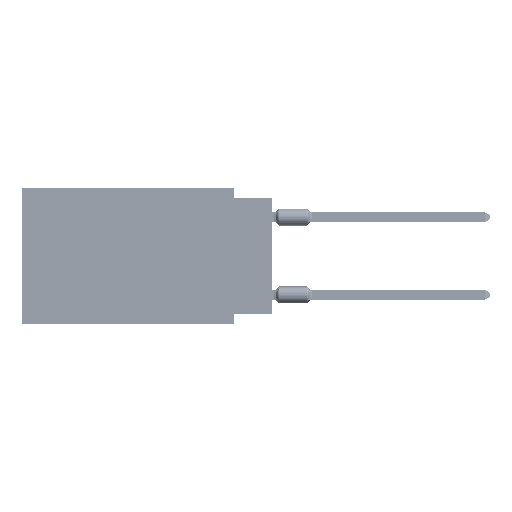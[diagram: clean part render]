
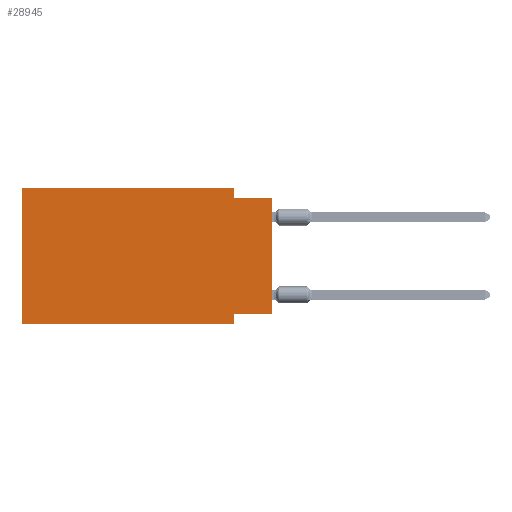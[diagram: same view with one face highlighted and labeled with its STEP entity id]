
A CAD part, left-side view. The second image highlights one B-rep face of the part: STEP entity #28945.
In plain terms, the highlighted planar face has unit normal (-1, 0, 0).
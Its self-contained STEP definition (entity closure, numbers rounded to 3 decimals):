
#859 = FACE_OUTER_BOUND ( 'NONE', #63787, .T. ) ;
#2923 = CARTESIAN_POINT ( 'NONE',  ( 0., 0., -8.255 ) ) ;
#4241 = EDGE_CURVE ( 'NONE', #46899, #16961, #41507, .T. ) ;
#4264 = LINE ( 'NONE', #56788, #30928 ) ;
#4663 = VECTOR ( 'NONE', #31019, 1000. ) ;
#4807 = CARTESIAN_POINT ( 'NONE',  ( 0., 0., -8.255 ) ) ;
#5105 = CARTESIAN_POINT ( 'NONE',  ( 0., 0., -0.635 ) ) ;
#5381 = CARTESIAN_POINT ( 'NONE',  ( 0., 0., 0. ) ) ;
#9938 = VERTEX_POINT ( 'NONE', #48765 ) ;
#11227 = LINE ( 'NONE', #5381, #59317 ) ;
#12024 = VERTEX_POINT ( 'NONE', #26387 ) ;
#13480 = DIRECTION ( 'NONE',  ( 0., -1., 0. ) ) ;
#13601 = ORIENTED_EDGE ( 'NONE', *, *, #71519, .T. ) ;
#14333 = VECTOR ( 'NONE', #43107, 1000. ) ;
#14846 = VECTOR ( 'NONE', #13480, 1000. ) ;
#16961 = VERTEX_POINT ( 'NONE', #5105 ) ;
#18136 = LINE ( 'NONE', #59744, #58381 ) ;
#18648 = VERTEX_POINT ( 'NONE', #25229 ) ;
#19322 = CARTESIAN_POINT ( 'NONE',  ( 0., 0., -0.635 ) ) ;
#19661 = VECTOR ( 'NONE', #68702, 1000. ) ;
#21537 = VERTEX_POINT ( 'NONE', #2923 ) ;
#23590 = DIRECTION ( 'NONE',  ( 0., 0., 1. ) ) ;
#23754 = EDGE_CURVE ( 'NONE', #74258, #9938, #4264, .T. ) ;
#24216 = CARTESIAN_POINT ( 'NONE',  ( 0., 16.383, 0. ) ) ;
#24217 = VERTEX_POINT ( 'NONE', #26371 ) ;
#24594 = PLANE ( 'NONE',  #66621 ) ;
#25229 = CARTESIAN_POINT ( 'NONE',  ( 0., 2.54, 0. ) ) ;
#26371 = CARTESIAN_POINT ( 'NONE',  ( 0., 16.383, 0. ) ) ;
#26387 = CARTESIAN_POINT ( 'NONE',  ( 0., 2.54, -8.255 ) ) ;
#28088 = ORIENTED_EDGE ( 'NONE', *, *, #75184, .F. ) ;
#28945 = ADVANCED_FACE ( 'NONE', ( #859 ), #24594, .F. ) ;
#29109 = DIRECTION ( 'NONE',  ( 0., 0., 1. ) ) ;
#30928 = VECTOR ( 'NONE', #51345, 1000. ) ;
#31019 = DIRECTION ( 'NONE',  ( 0., 0., -1. ) ) ;
#35337 = EDGE_CURVE ( 'NONE', #74258, #24217, #18136, .T. ) ;
#36049 = DIRECTION ( 'NONE',  ( 0., -1., 0. ) ) ;
#37648 = CARTESIAN_POINT ( 'NONE',  ( 0., 2.54, 0. ) ) ;
#38296 = ORIENTED_EDGE ( 'NONE', *, *, #71605, .F. ) ;
#38905 = CARTESIAN_POINT ( 'NONE',  ( 0., 16.383, -8.89 ) ) ;
#41507 = LINE ( 'NONE', #19322, #53825 ) ;
#43035 = LINE ( 'NONE', #66757, #14846 ) ;
#43107 = DIRECTION ( 'NONE',  ( 0., 0., -1. ) ) ;
#45777 = EDGE_CURVE ( 'NONE', #21537, #12024, #50836, .T. ) ;
#46899 = VERTEX_POINT ( 'NONE', #66030 ) ;
#48246 = ORIENTED_EDGE ( 'NONE', *, *, #4241, .F. ) ;
#48325 = DIRECTION ( 'NONE',  ( 1., 0., 0. ) ) ;
#48765 = CARTESIAN_POINT ( 'NONE',  ( 0., 2.54, -8.89 ) ) ;
#48957 = CARTESIAN_POINT ( 'NONE',  ( 0., 2.54, -8.89 ) ) ;
#50836 = LINE ( 'NONE', #4807, #19661 ) ;
#51345 = DIRECTION ( 'NONE',  ( 0., -1., 0. ) ) ;
#53825 = VECTOR ( 'NONE', #36049, 1000. ) ;
#56788 = CARTESIAN_POINT ( 'NONE',  ( 0., 16.383, -8.89 ) ) ;
#58381 = VECTOR ( 'NONE', #23590, 1000. ) ;
#58649 = EDGE_CURVE ( 'NONE', #12024, #9938, #72659, .T. ) ;
#59317 = VECTOR ( 'NONE', #29109, 1000. ) ;
#59744 = CARTESIAN_POINT ( 'NONE',  ( 0., 16.383, 0. ) ) ;
#62369 = ORIENTED_EDGE ( 'NONE', *, *, #58649, .F. ) ;
#63787 = EDGE_LOOP ( 'NONE', ( #13601, #48246, #38296, #28088, #71480, #74893, #62369, #69459 ) ) ;
#66030 = CARTESIAN_POINT ( 'NONE',  ( 0., 2.54, -0.635 ) ) ;
#66621 = AXIS2_PLACEMENT_3D ( 'NONE', #24216, #48325, #72421 ) ;
#66757 = CARTESIAN_POINT ( 'NONE',  ( 0., 16.383, 0. ) ) ;
#68702 = DIRECTION ( 'NONE',  ( 0., 1., 0. ) ) ;
#69459 = ORIENTED_EDGE ( 'NONE', *, *, #45777, .F. ) ;
#71480 = ORIENTED_EDGE ( 'NONE', *, *, #35337, .F. ) ;
#71519 = EDGE_CURVE ( 'NONE', #21537, #16961, #11227, .T. ) ;
#71605 = EDGE_CURVE ( 'NONE', #18648, #46899, #72636, .T. ) ;
#72421 = DIRECTION ( 'NONE',  ( 0., 0., -1. ) ) ;
#72636 = LINE ( 'NONE', #37648, #4663 ) ;
#72659 = LINE ( 'NONE', #48957, #14333 ) ;
#74258 = VERTEX_POINT ( 'NONE', #38905 ) ;
#74893 = ORIENTED_EDGE ( 'NONE', *, *, #23754, .T. ) ;
#75184 = EDGE_CURVE ( 'NONE', #24217, #18648, #43035, .T. ) ;
